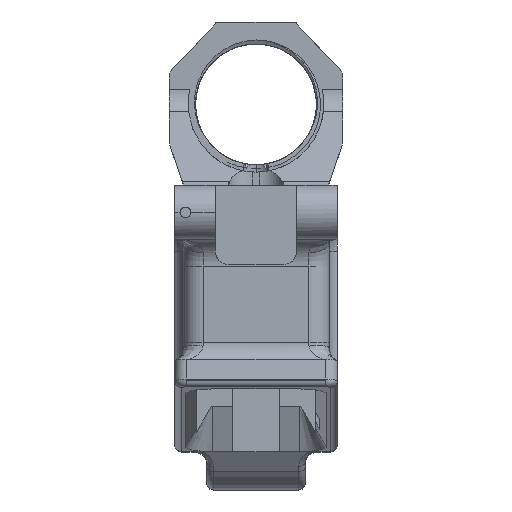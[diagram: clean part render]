
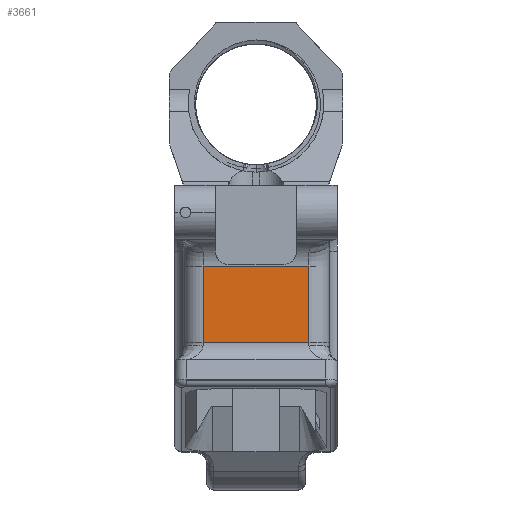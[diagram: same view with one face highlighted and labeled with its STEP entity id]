
A CAD part, top view. The second image highlights one B-rep face of the part: STEP entity #3661.
In plain terms, the highlighted planar face has unit normal (0, 0, 1).
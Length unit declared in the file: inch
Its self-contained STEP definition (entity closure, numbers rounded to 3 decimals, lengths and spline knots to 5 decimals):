
#48 = CARTESIAN_POINT ( 'NONE',  ( -0.488, -0.74479, 8.542 ) ) ;
#79 = CARTESIAN_POINT ( 'NONE',  ( 0.8, -0.74479, 8.542 ) ) ;
#288 = ORIENTED_EDGE ( 'NONE', *, *, #10334, .T. ) ;
#595 = VERTEX_POINT ( 'NONE', #9506 ) ;
#1018 = CARTESIAN_POINT ( 'NONE',  ( -0.488, -1.45201, 8.542 ) ) ;
#1351 = CARTESIAN_POINT ( 'NONE',  ( 0.8, -1.45201, 8.542 ) ) ;
#1462 = FACE_OUTER_BOUND ( 'NONE', #9428, .T. ) ;
#1886 = LINE ( 'NONE', #16490, #16131 ) ;
#1890 = PLANE ( 'NONE',  #3442 ) ;
#2382 = LINE ( 'NONE', #79, #16650 ) ;
#3135 = VERTEX_POINT ( 'NONE', #48 ) ;
#3296 = DIRECTION ( 'NONE',  ( 0., 1., 0. ) ) ;
#3442 = AXIS2_PLACEMENT_3D ( 'NONE', #6002, #11579, #3296 ) ;
#3444 = EDGE_CURVE ( 'NONE', #595, #12287, #7746, .T. ) ;
#3661 = ADVANCED_FACE ( 'NONE', ( #1462 ), #1890, .F. ) ;
#5188 = DIRECTION ( 'NONE',  ( 0., -1., 0. ) ) ;
#6002 = CARTESIAN_POINT ( 'NONE',  ( 0.8, -1.61392, 8.542 ) ) ;
#6619 = CARTESIAN_POINT ( 'NONE',  ( 0.488, -1.45201, 8.542 ) ) ;
#6758 = EDGE_CURVE ( 'NONE', #12287, #16773, #1886, .T. ) ;
#7319 = VECTOR ( 'NONE', #15132, 39.37008 ) ;
#7746 = LINE ( 'NONE', #1351, #7319 ) ;
#8356 = DIRECTION ( 'NONE',  ( -1., 0., 0. ) ) ;
#8439 = CARTESIAN_POINT ( 'NONE',  ( 0.488, -0.74479, 8.542 ) ) ;
#9428 = EDGE_LOOP ( 'NONE', ( #16877, #15820, #10173, #288 ) ) ;
#9506 = CARTESIAN_POINT ( 'NONE',  ( -0.488, -1.45201, 8.542 ) ) ;
#10173 = ORIENTED_EDGE ( 'NONE', *, *, #17196, .T. ) ;
#10334 = EDGE_CURVE ( 'NONE', #3135, #595, #12828, .T. ) ;
#11579 = DIRECTION ( 'NONE',  ( 0., 0., -1. ) ) ;
#12287 = VERTEX_POINT ( 'NONE', #6619 ) ;
#12344 = DIRECTION ( 'NONE',  ( 0., 1., 0. ) ) ;
#12828 = LINE ( 'NONE', #1018, #16019 ) ;
#15132 = DIRECTION ( 'NONE',  ( 1., 0., 0. ) ) ;
#15820 = ORIENTED_EDGE ( 'NONE', *, *, #6758, .T. ) ;
#16019 = VECTOR ( 'NONE', #5188, 39.37008 ) ;
#16131 = VECTOR ( 'NONE', #12344, 39.37008 ) ;
#16490 = CARTESIAN_POINT ( 'NONE',  ( 0.488, -0.74479, 8.542 ) ) ;
#16650 = VECTOR ( 'NONE', #8356, 39.37008 ) ;
#16773 = VERTEX_POINT ( 'NONE', #8439 ) ;
#16877 = ORIENTED_EDGE ( 'NONE', *, *, #3444, .T. ) ;
#17196 = EDGE_CURVE ( 'NONE', #16773, #3135, #2382, .T. ) ;
